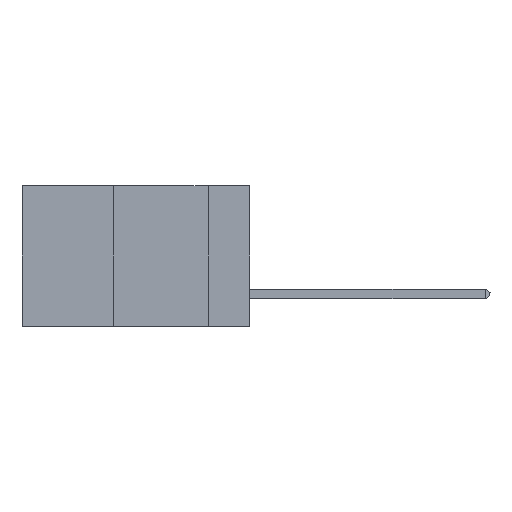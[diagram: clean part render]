
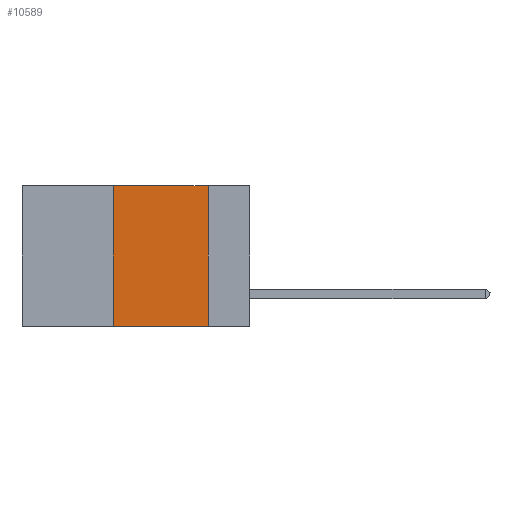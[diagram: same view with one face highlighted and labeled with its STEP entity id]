
A CAD part, left-side view. The second image highlights one B-rep face of the part: STEP entity #10589.
In plain terms, the highlighted planar face has unit normal (-1, 0, 0).
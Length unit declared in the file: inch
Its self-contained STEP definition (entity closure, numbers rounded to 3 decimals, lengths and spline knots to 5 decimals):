
#2886 = VECTOR ( 'NONE', #12480, 39.37008 ) ;
#2916 = AXIS2_PLACEMENT_3D ( 'NONE', #6336, #11931, #11737 ) ;
#3007 = CARTESIAN_POINT ( 'NONE',  ( 0., 0.36, 0. ) ) ;
#3135 = ORIENTED_EDGE ( 'NONE', *, *, #9268, .F. ) ;
#3280 = DIRECTION ( 'NONE',  ( 0., -1., 0. ) ) ;
#3754 = VECTOR ( 'NONE', #4611, 39.37008 ) ;
#4611 = DIRECTION ( 'NONE',  ( 0., -1., 0. ) ) ;
#5238 = LINE ( 'NONE', #13029, #3754 ) ;
#5517 = CARTESIAN_POINT ( 'NONE',  ( 0., 0.11, 0. ) ) ;
#6336 = CARTESIAN_POINT ( 'NONE',  ( 0., 0.6, 0. ) ) ;
#6368 = VERTEX_POINT ( 'NONE', #12788 ) ;
#6793 = CARTESIAN_POINT ( 'NONE',  ( 0., 0.11, 0. ) ) ;
#7271 = CARTESIAN_POINT ( 'NONE',  ( 0., 0.6, -0.37 ) ) ;
#7287 = LINE ( 'NONE', #17354, #15235 ) ;
#7598 = VECTOR ( 'NONE', #3280, 39.37008 ) ;
#8158 = VERTEX_POINT ( 'NONE', #10250 ) ;
#9110 = PLANE ( 'NONE',  #2916 ) ;
#9268 = EDGE_CURVE ( 'NONE', #9331, #8158, #12941, .T. ) ;
#9331 = VERTEX_POINT ( 'NONE', #5517 ) ;
#9346 = EDGE_LOOP ( 'NONE', ( #3135, #17414, #15733, #13582 ) ) ;
#9378 = FACE_OUTER_BOUND ( 'NONE', #9346, .T. ) ;
#10250 = CARTESIAN_POINT ( 'NONE',  ( 0., 0.11, -0.37 ) ) ;
#10269 = DIRECTION ( 'NONE',  ( 0., 0., 1. ) ) ;
#10589 = ADVANCED_FACE ( 'NONE', ( #9378 ), #9110, .F. ) ;
#11451 = EDGE_CURVE ( 'NONE', #17835, #9331, #5238, .T. ) ;
#11737 = DIRECTION ( 'NONE',  ( 0., 0., -1. ) ) ;
#11931 = DIRECTION ( 'NONE',  ( 1., 0., 0. ) ) ;
#12480 = DIRECTION ( 'NONE',  ( 0., 0., -1. ) ) ;
#12788 = CARTESIAN_POINT ( 'NONE',  ( 0., 0.36, -0.37 ) ) ;
#12941 = LINE ( 'NONE', #6793, #2886 ) ;
#13029 = CARTESIAN_POINT ( 'NONE',  ( 0., 0.6, 0. ) ) ;
#13469 = EDGE_CURVE ( 'NONE', #6368, #8158, #16400, .T. ) ;
#13582 = ORIENTED_EDGE ( 'NONE', *, *, #13469, .T. ) ;
#15235 = VECTOR ( 'NONE', #10269, 39.37008 ) ;
#15345 = EDGE_CURVE ( 'NONE', #6368, #17835, #7287, .T. ) ;
#15733 = ORIENTED_EDGE ( 'NONE', *, *, #15345, .F. ) ;
#16400 = LINE ( 'NONE', #7271, #7598 ) ;
#17354 = CARTESIAN_POINT ( 'NONE',  ( 0., 0.36, 0. ) ) ;
#17414 = ORIENTED_EDGE ( 'NONE', *, *, #11451, .F. ) ;
#17835 = VERTEX_POINT ( 'NONE', #3007 ) ;
